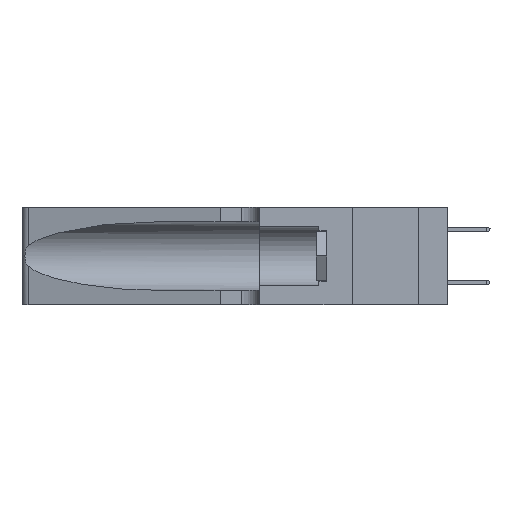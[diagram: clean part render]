
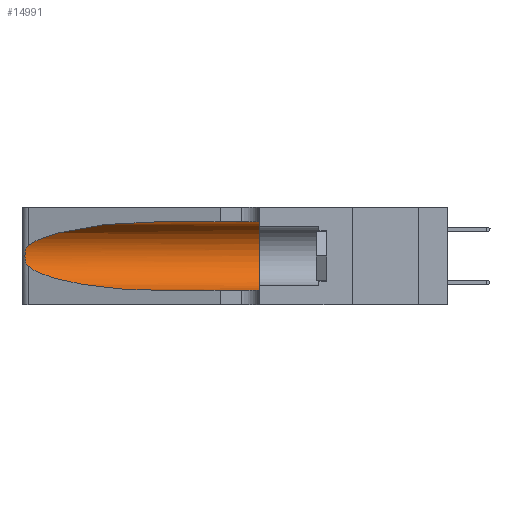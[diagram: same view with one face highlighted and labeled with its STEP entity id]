
A CAD part, left-side view. The second image highlights one B-rep face of the part: STEP entity #14991.
In plain terms, the highlighted cylindrical face has radius 3.308 mm (diameter 6.617 mm), a partial arc.
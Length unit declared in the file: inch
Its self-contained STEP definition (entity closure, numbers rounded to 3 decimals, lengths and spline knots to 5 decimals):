
#404 = EDGE_CURVE ( 'NONE', #8557, #34930, #21403, .T. ) ;
#1308 = DIRECTION ( 'NONE',  ( 0., -1., 0. ) ) ;
#1434 = EDGE_CURVE ( 'NONE', #2299, #26027, #25294, .T. ) ;
#2299 = VERTEX_POINT ( 'NONE', #7630 ) ;
#3513 = CARTESIAN_POINT ( 'NONE',  ( 0.25555, 1.22993, 0.14849 ) ) ;
#3693 = EDGE_CURVE ( 'NONE', #20420, #8557, #41517, .T. ) ;
#3702 = VERTEX_POINT ( 'NONE', #8447 ) ;
#4392 = ORIENTED_EDGE ( 'NONE', *, *, #43248, .T. ) ;
#4536 = VECTOR ( 'NONE', #1308, 39.37008 ) ;
#6563 = CARTESIAN_POINT ( 'NONE',  ( 0.1305, 0.35, 0.05475 ) ) ;
#7630 = CARTESIAN_POINT ( 'NONE',  ( 0.25487, 1.22718, 0.22369 ) ) ;
#8447 = CARTESIAN_POINT ( 'NONE',  ( 0.1305, 0.72297, 0.05475 ) ) ;
#8557 = VERTEX_POINT ( 'NONE', #29039 ) ;
#9681 = CARTESIAN_POINT ( 'NONE',  ( 0.18966, 0.96281, 0.31525 ) ) ;
#9750 = CARTESIAN_POINT ( 'NONE',  ( 0.18966, 0.96281, 0.05475 ) ) ;
#10467 = CARTESIAN_POINT ( 'NONE',  ( 0.25787, 1.23484, 0.2124 ) ) ;
#10689 = CYLINDRICAL_SURFACE ( 'NONE', #22605, 0.13025 ) ;
#10986 = DIRECTION ( 'NONE',  ( 0., -1., 0. ) ) ;
#11773 = FACE_OUTER_BOUND ( 'NONE', #40352, .T. ) ;
#14001 = CARTESIAN_POINT ( 'NONE',  ( 0.26018, 1.23835, 0.19895 ) ) ;
#14381 = CARTESIAN_POINT ( 'NONE',  ( 0.1305, 1.61858, 0.185 ) ) ;
#14991 = ADVANCED_FACE ( 'NONE', ( #11773 ), #10689, .F. ) ;
#17356 = CARTESIAN_POINT ( 'NONE',  ( 0.1305, 0.35, 0.185 ) ) ;
#17561 = CARTESIAN_POINT ( 'NONE',  ( 0.26075, 1.23896, 0.178 ) ) ;
#17645 = ORIENTED_EDGE ( 'NONE', *, *, #22228, .T. ) ;
#18610 =( BOUNDED_CURVE ( )  B_SPLINE_CURVE ( 3, ( #44275, #20207, #9750, #34065 ),
 .UNSPECIFIED., .F., .T. ) 
 B_SPLINE_CURVE_WITH_KNOTS ( ( 4, 4 ),
 ( 3.44316, 4.71239 ),
 .UNSPECIFIED. ) 
 CURVE ( )  GEOMETRIC_REPRESENTATION_ITEM ( )  RATIONAL_B_SPLINE_CURVE ( ( 1., 0.87, 0.87, 1. ) ) 
 REPRESENTATION_ITEM ( '' )  );
#19227 = AXIS2_PLACEMENT_3D ( 'NONE', #17356, #41479, #20878 ) ;
#20207 = CARTESIAN_POINT ( 'NONE',  ( 0.2373, 1.15595, 0.08982 ) ) ;
#20281 = CARTESIAN_POINT ( 'NONE',  ( 0.2373, 1.15595, 0.28018 ) ) ;
#20420 = VERTEX_POINT ( 'NONE', #38781 ) ;
#20878 = DIRECTION ( 'NONE',  ( 0., 0., 1. ) ) ;
#21074 = CARTESIAN_POINT ( 'NONE',  ( 0.25856, 1.23593, 0.16098 ) ) ;
#21403 = CIRCLE ( 'NONE', #19227, 0.13025 ) ;
#21966 =( BOUNDED_CURVE ( )  B_SPLINE_CURVE ( 3, ( #40602, #9681, #20281, #44357 ),
 .UNSPECIFIED., .F., .T. ) 
 B_SPLINE_CURVE_WITH_KNOTS ( ( 4, 4 ),
 ( 1.5708, 2.84003 ),
 .UNSPECIFIED. ) 
 CURVE ( )  GEOMETRIC_REPRESENTATION_ITEM ( )  RATIONAL_B_SPLINE_CURVE ( ( 1., 0.87, 0.87, 1. ) ) 
 REPRESENTATION_ITEM ( '' )  );
#22228 = EDGE_CURVE ( 'NONE', #20420, #2299, #21966, .T. ) ;
#22412 = CARTESIAN_POINT ( 'NONE',  ( 0.1305, 1.61858, 0.31525 ) ) ;
#22605 = AXIS2_PLACEMENT_3D ( 'NONE', #14381, #10986, #35276 ) ;
#22694 = LINE ( 'NONE', #28814, #39886 ) ;
#24543 = CARTESIAN_POINT ( 'NONE',  ( 0.25639, 1.23186, 0.15144 ) ) ;
#25294 = B_SPLINE_CURVE_WITH_KNOTS ( 'NONE', 3,
 ( #31314, #27848, #38060, #10467, #34764, #14001, #38206, #17561, #41671, #21074, #34111, #24543, #3513, #27999 ),
 .UNSPECIFIED., .F., .F.,
 ( 4, 2, 2, 2, 2, 2, 4 ),
 ( 0., 0.00027, 0.00053, 0.00107, 0.0016, 0.00187, 0.00214 ),
 .UNSPECIFIED. ) ;
#26027 = VERTEX_POINT ( 'NONE', #33165 ) ;
#27848 = CARTESIAN_POINT ( 'NONE',  ( 0.25555, 1.22994, 0.2215 ) ) ;
#27999 = CARTESIAN_POINT ( 'NONE',  ( 0.25487, 1.22718, 0.14631 ) ) ;
#28814 = CARTESIAN_POINT ( 'NONE',  ( 0.1305, 1.61858, 0.05475 ) ) ;
#29039 = CARTESIAN_POINT ( 'NONE',  ( 0.1305, 0.35, 0.31525 ) ) ;
#31314 = CARTESIAN_POINT ( 'NONE',  ( 0.25487, 1.22718, 0.22369 ) ) ;
#32260 = ORIENTED_EDGE ( 'NONE', *, *, #33270, .T. ) ;
#33165 = CARTESIAN_POINT ( 'NONE',  ( 0.25487, 1.22718, 0.14631 ) ) ;
#33270 = EDGE_CURVE ( 'NONE', #3702, #34930, #22694, .T. ) ;
#34065 = CARTESIAN_POINT ( 'NONE',  ( 0.1305, 0.72297, 0.05475 ) ) ;
#34111 = CARTESIAN_POINT ( 'NONE',  ( 0.25789, 1.23486, 0.15765 ) ) ;
#34764 = CARTESIAN_POINT ( 'NONE',  ( 0.25854, 1.2359, 0.20912 ) ) ;
#34930 = VERTEX_POINT ( 'NONE', #6563 ) ;
#35276 = DIRECTION ( 'NONE',  ( 0., 0., -1. ) ) ;
#35475 = ORIENTED_EDGE ( 'NONE', *, *, #404, .F. ) ;
#38060 = CARTESIAN_POINT ( 'NONE',  ( 0.25639, 1.23184, 0.21858 ) ) ;
#38144 = ORIENTED_EDGE ( 'NONE', *, *, #1434, .T. ) ;
#38206 = CARTESIAN_POINT ( 'NONE',  ( 0.26075, 1.23896, 0.19203 ) ) ;
#38781 = CARTESIAN_POINT ( 'NONE',  ( 0.1305, 0.72297, 0.31525 ) ) ;
#39886 = VECTOR ( 'NONE', #42499, 39.37008 ) ;
#40352 = EDGE_LOOP ( 'NONE', ( #17645, #38144, #4392, #32260, #35475, #44612 ) ) ;
#40602 = CARTESIAN_POINT ( 'NONE',  ( 0.1305, 0.72297, 0.31525 ) ) ;
#41479 = DIRECTION ( 'NONE',  ( 0., 1., 0. ) ) ;
#41517 = LINE ( 'NONE', #22412, #4536 ) ;
#41671 = CARTESIAN_POINT ( 'NONE',  ( 0.26017, 1.23833, 0.17102 ) ) ;
#42499 = DIRECTION ( 'NONE',  ( 0., -1., 0. ) ) ;
#43248 = EDGE_CURVE ( 'NONE', #26027, #3702, #18610, .T. ) ;
#44275 = CARTESIAN_POINT ( 'NONE',  ( 0.25487, 1.22718, 0.14631 ) ) ;
#44357 = CARTESIAN_POINT ( 'NONE',  ( 0.25487, 1.22718, 0.22369 ) ) ;
#44612 = ORIENTED_EDGE ( 'NONE', *, *, #3693, .F. ) ;
